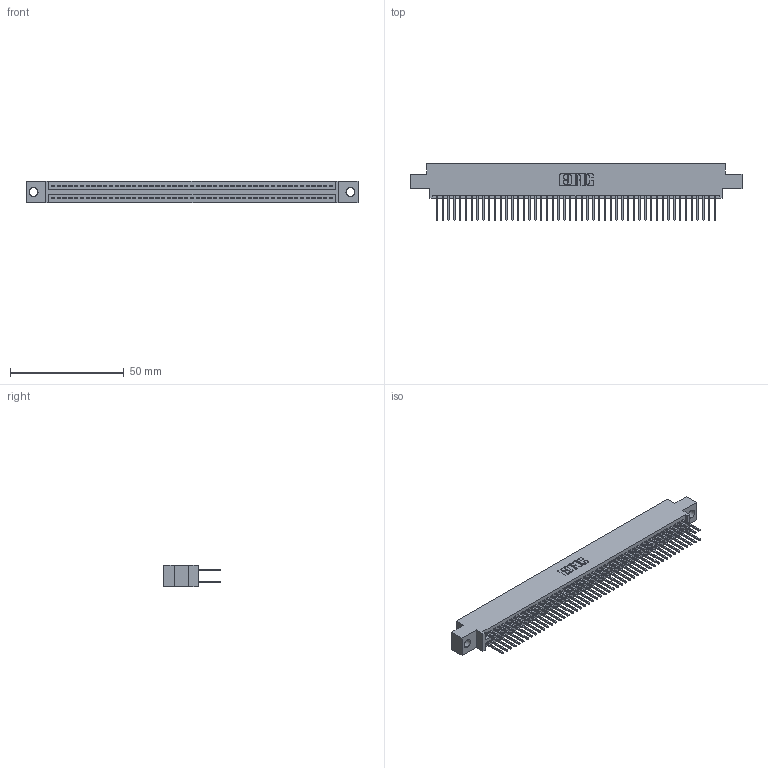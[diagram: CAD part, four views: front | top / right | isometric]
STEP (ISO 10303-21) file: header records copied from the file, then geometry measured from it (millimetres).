
FILE_DESCRIPTION (( 'STEP AP203' ), '1' );
FILE_NAME ('395-098-523-804.STEP', '2021-06-17T12:38:39', ( '' ), ( '' ), 'SwSTEP 2.0', 'SolidWorks 2020', '' );
FILE_SCHEMA (( 'CONFIG_CONTROL_DESIGN' ));
Length unit declared in the file: inch
Products named in the file (3): 345 Part_0.170 Offset - 0.156 Dia-TI; 345-292-001_345-293-123; 395-098-523-804
Assembly tree (99 placements, depth 2):
  395-098-523-804
    345 Part_0.170 Offset - 0.156 Dia-TI
    345-292-001_345-293-123  x98
Bounding box: 145.67 x 24.82 x 9.4 mm (x, y, z)
Volume: 14197 mm3; surface area: 22017.1 mm2
Topology: 99 solids, 99 shells, 5044 faces, 14991 edges, 9862 vertices
Faces by surface type: plane 3332, cylinder 1712
Entity records: 38073 total; most frequent: CARTESIAN_POINT 6382, ORIENTED_EDGE 6314, DIRECTION 5617, EDGE_CURVE 3157, VECTOR 2829, LINE 2829, VERTEX_POINT 2102, AXIS2_PLACEMENT_3D 1394
